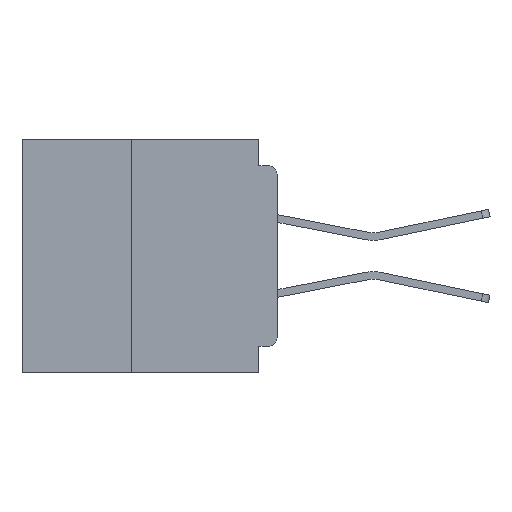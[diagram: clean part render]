
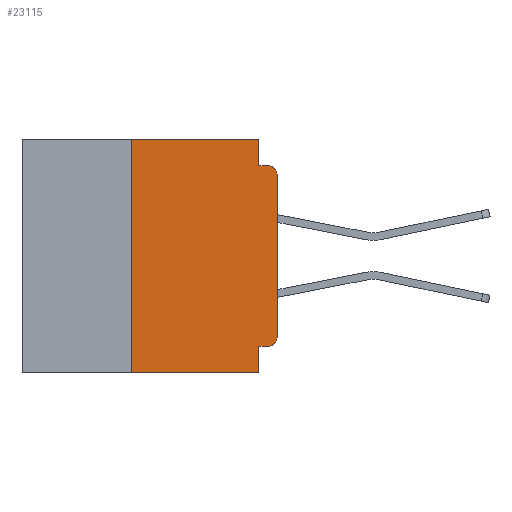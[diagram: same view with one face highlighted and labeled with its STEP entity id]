
A CAD part, left-side view. The second image highlights one B-rep face of the part: STEP entity #23115.
In plain terms, the highlighted planar face has unit normal (-1, 0, 0).
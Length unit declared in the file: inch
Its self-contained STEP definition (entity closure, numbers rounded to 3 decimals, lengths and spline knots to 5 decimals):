
#150 = VERTEX_POINT ( 'NONE', #25606 ) ;
#770 = FACE_OUTER_BOUND ( 'NONE', #34748, .T. ) ;
#825 = ORIENTED_EDGE ( 'NONE', *, *, #10734, .F. ) ;
#2071 = VERTEX_POINT ( 'NONE', #28040 ) ;
#3031 = VECTOR ( 'NONE', #20050, 39.37008 ) ;
#3371 = VECTOR ( 'NONE', #5678, 39.37008 ) ;
#3663 = CARTESIAN_POINT ( 'NONE',  ( 0., 0.25, -0.4 ) ) ;
#3866 = CARTESIAN_POINT ( 'NONE',  ( 0., 0., -0.06 ) ) ;
#3967 = EDGE_CURVE ( 'NONE', #12188, #22284, #13133, .T. ) ;
#4035 = ORIENTED_EDGE ( 'NONE', *, *, #24400, .F. ) ;
#4199 = EDGE_CURVE ( 'NONE', #22284, #30536, #6088, .T. ) ;
#4425 = DIRECTION ( 'NONE',  ( 0., 1., 0. ) ) ;
#5196 = ORIENTED_EDGE ( 'NONE', *, *, #27423, .F. ) ;
#5283 = AXIS2_PLACEMENT_3D ( 'NONE', #17586, #17577, #17539 ) ;
#5669 = LINE ( 'NONE', #20724, #17971 ) ;
#5678 = DIRECTION ( 'NONE',  ( 0., -1., 0. ) ) ;
#6088 = CIRCLE ( 'NONE', #5283, 0.015 ) ;
#6413 = CARTESIAN_POINT ( 'NONE',  ( 0., 0.015, -0.355 ) ) ;
#7176 = LINE ( 'NONE', #30862, #28431 ) ;
#7361 = ORIENTED_EDGE ( 'NONE', *, *, #23603, .T. ) ;
#7434 = CIRCLE ( 'NONE', #32594, 0.015 ) ;
#8283 = DIRECTION ( 'NONE',  ( 1., 0., 0. ) ) ;
#9023 = LINE ( 'NONE', #30107, #17329 ) ;
#9435 = CARTESIAN_POINT ( 'NONE',  ( 0., 0., -0.34 ) ) ;
#9754 = CARTESIAN_POINT ( 'NONE',  ( 0., 0.031, 0. ) ) ;
#9937 = VERTEX_POINT ( 'NONE', #3663 ) ;
#10571 = LINE ( 'NONE', #17153, #3031 ) ;
#10734 = EDGE_CURVE ( 'NONE', #24080, #150, #9023, .T. ) ;
#10911 = LINE ( 'NONE', #27468, #3371 ) ;
#12188 = VERTEX_POINT ( 'NONE', #9435 ) ;
#13133 = LINE ( 'NONE', #21927, #35800 ) ;
#13299 = VERTEX_POINT ( 'NONE', #9754 ) ;
#14091 = VECTOR ( 'NONE', #26732, 39.37008 ) ;
#14489 = EDGE_CURVE ( 'NONE', #9937, #150, #5669, .T. ) ;
#14966 = AXIS2_PLACEMENT_3D ( 'NONE', #19405, #8283, #27684 ) ;
#14993 = LINE ( 'NONE', #23981, #14091 ) ;
#16113 = DIRECTION ( 'NONE',  ( -1., 0., 0. ) ) ;
#16358 = ORIENTED_EDGE ( 'NONE', *, *, #4199, .T. ) ;
#16482 = DIRECTION ( 'NONE',  ( 0., 0., -1. ) ) ;
#16913 = ORIENTED_EDGE ( 'NONE', *, *, #3967, .T. ) ;
#17153 = CARTESIAN_POINT ( 'NONE',  ( 0., 0.031, 0. ) ) ;
#17329 = VECTOR ( 'NONE', #16482, 39.37008 ) ;
#17539 = DIRECTION ( 'NONE',  ( 0., 0., -1. ) ) ;
#17577 = DIRECTION ( 'NONE',  ( -1., 0., 0. ) ) ;
#17586 = CARTESIAN_POINT ( 'NONE',  ( 0., 0.015, -0.06 ) ) ;
#17971 = VECTOR ( 'NONE', #17973, 39.37008 ) ;
#17973 = DIRECTION ( 'NONE',  ( 0., -1., 0. ) ) ;
#18336 = ORIENTED_EDGE ( 'NONE', *, *, #24777, .F. ) ;
#19062 = ORIENTED_EDGE ( 'NONE', *, *, #34647, .F. ) ;
#19405 = CARTESIAN_POINT ( 'NONE',  ( 0., 0.437, 0. ) ) ;
#20050 = DIRECTION ( 'NONE',  ( 0., 0., -1. ) ) ;
#20724 = CARTESIAN_POINT ( 'NONE',  ( 0., 0.437, -0.4 ) ) ;
#21177 = CARTESIAN_POINT ( 'NONE',  ( 0., 0., -0.355 ) ) ;
#21927 = CARTESIAN_POINT ( 'NONE',  ( 0., 0., 0. ) ) ;
#21973 = DIRECTION ( 'NONE',  ( 0., 0., 1. ) ) ;
#22284 = VERTEX_POINT ( 'NONE', #3866 ) ;
#23115 = ADVANCED_FACE ( 'NONE', ( #770 ), #24830, .F. ) ;
#23603 = EDGE_CURVE ( 'NONE', #32704, #12188, #7434, .T. ) ;
#23981 = CARTESIAN_POINT ( 'NONE',  ( 0., 0., -0.045 ) ) ;
#24080 = VERTEX_POINT ( 'NONE', #31732 ) ;
#24400 = EDGE_CURVE ( 'NONE', #34205, #13299, #10911, .T. ) ;
#24777 = EDGE_CURVE ( 'NONE', #32704, #24080, #33629, .T. ) ;
#24830 = PLANE ( 'NONE',  #14966 ) ;
#25606 = CARTESIAN_POINT ( 'NONE',  ( 0., 0.031, -0.4 ) ) ;
#26043 = ORIENTED_EDGE ( 'NONE', *, *, #29524, .F. ) ;
#26232 = CARTESIAN_POINT ( 'NONE',  ( 0., 0.25, 0. ) ) ;
#26732 = DIRECTION ( 'NONE',  ( 0., -1., 0. ) ) ;
#27423 = EDGE_CURVE ( 'NONE', #9937, #34205, #7176, .T. ) ;
#27468 = CARTESIAN_POINT ( 'NONE',  ( 0., 0.437, 0. ) ) ;
#27684 = DIRECTION ( 'NONE',  ( 0., 0., -1. ) ) ;
#28040 = CARTESIAN_POINT ( 'NONE',  ( 0., 0.031, -0.045 ) ) ;
#28186 = VECTOR ( 'NONE', #4425, 39.37008 ) ;
#28431 = VECTOR ( 'NONE', #33561, 39.37008 ) ;
#29524 = EDGE_CURVE ( 'NONE', #2071, #30536, #14993, .T. ) ;
#30107 = CARTESIAN_POINT ( 'NONE',  ( 0., 0.031, -0.4 ) ) ;
#30536 = VERTEX_POINT ( 'NONE', #34948 ) ;
#30862 = CARTESIAN_POINT ( 'NONE',  ( 0., 0.25, -0.4 ) ) ;
#31732 = CARTESIAN_POINT ( 'NONE',  ( 0., 0.031, -0.355 ) ) ;
#32450 = CARTESIAN_POINT ( 'NONE',  ( 0., 0.015, -0.34 ) ) ;
#32594 = AXIS2_PLACEMENT_3D ( 'NONE', #32450, #16113, #35143 ) ;
#32704 = VERTEX_POINT ( 'NONE', #6413 ) ;
#33561 = DIRECTION ( 'NONE',  ( 0., 0., 1. ) ) ;
#33629 = LINE ( 'NONE', #21177, #28186 ) ;
#34205 = VERTEX_POINT ( 'NONE', #26232 ) ;
#34647 = EDGE_CURVE ( 'NONE', #13299, #2071, #10571, .T. ) ;
#34748 = EDGE_LOOP ( 'NONE', ( #16913, #16358, #26043, #19062, #4035, #5196, #35412, #825, #18336, #7361 ) ) ;
#34948 = CARTESIAN_POINT ( 'NONE',  ( 0., 0.015, -0.045 ) ) ;
#35143 = DIRECTION ( 'NONE',  ( 0., 0., -1. ) ) ;
#35412 = ORIENTED_EDGE ( 'NONE', *, *, #14489, .T. ) ;
#35800 = VECTOR ( 'NONE', #21973, 39.37008 ) ;
